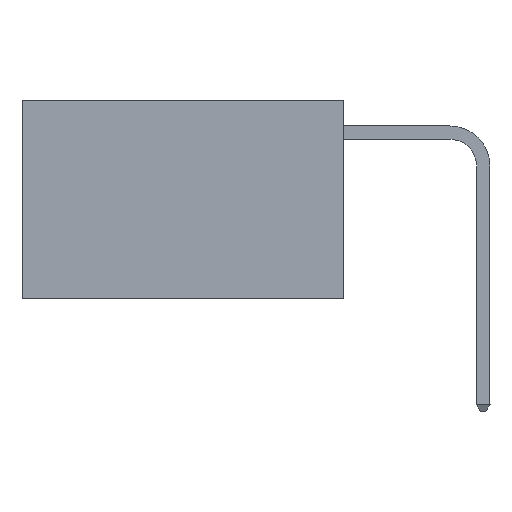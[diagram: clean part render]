
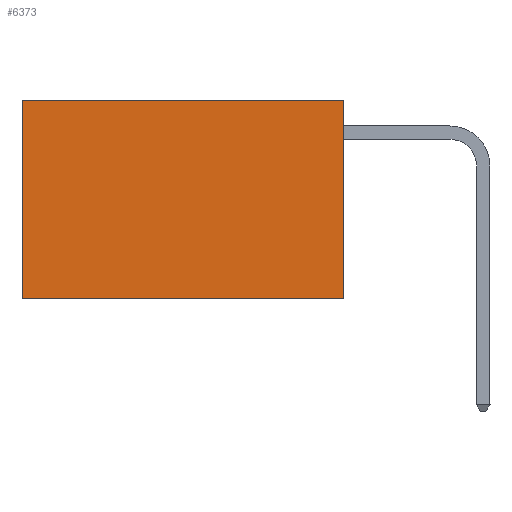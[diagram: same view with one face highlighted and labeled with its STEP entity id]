
A CAD part, left-side view. The second image highlights one B-rep face of the part: STEP entity #6373.
In plain terms, the highlighted planar face has unit normal (-1, 0, 0).
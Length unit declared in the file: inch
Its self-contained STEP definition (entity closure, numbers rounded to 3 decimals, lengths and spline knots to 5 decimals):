
#83 = ORIENTED_EDGE ( 'NONE', *, *, #4615, .T. ) ;
#137 = CARTESIAN_POINT ( 'NONE',  ( 0.2625, 0., 0. ) ) ;
#226 = CARTESIAN_POINT ( 'NONE',  ( 0.2625, 0.6, 0. ) ) ;
#648 = CARTESIAN_POINT ( 'NONE',  ( 0.2625, 0.6, 0. ) ) ;
#713 = DIRECTION ( 'NONE',  ( 0., 1., 0. ) ) ;
#1568 = DIRECTION ( 'NONE',  ( 0., 0., -1. ) ) ;
#1773 = CARTESIAN_POINT ( 'NONE',  ( 0.2625, 0., 0. ) ) ;
#3009 = AXIS2_PLACEMENT_3D ( 'NONE', #1773, #12237, #3211 ) ;
#3211 = DIRECTION ( 'NONE',  ( 0., 0., -1. ) ) ;
#3341 = LINE ( 'NONE', #137, #10021 ) ;
#4093 = VERTEX_POINT ( 'NONE', #15468 ) ;
#4615 = EDGE_CURVE ( 'NONE', #10963, #17523, #11749, .T. ) ;
#4798 = EDGE_CURVE ( 'NONE', #4093, #17523, #14006, .T. ) ;
#5026 = ORIENTED_EDGE ( 'NONE', *, *, #4798, .F. ) ;
#5235 = ORIENTED_EDGE ( 'NONE', *, *, #11759, .T. ) ;
#6373 = ADVANCED_FACE ( 'NONE', ( #18114 ), #16524, .F. ) ;
#6678 = ORIENTED_EDGE ( 'NONE', *, *, #17044, .F. ) ;
#6759 = VECTOR ( 'NONE', #1568, 39.37008 ) ;
#10021 = VECTOR ( 'NONE', #10690, 39.37008 ) ;
#10690 = DIRECTION ( 'NONE',  ( 0., 1., 0. ) ) ;
#10709 = CARTESIAN_POINT ( 'NONE',  ( 0.2625, 0., 0. ) ) ;
#10814 = VERTEX_POINT ( 'NONE', #17038 ) ;
#10963 = VERTEX_POINT ( 'NONE', #226 ) ;
#11062 = VECTOR ( 'NONE', #15085, 39.37008 ) ;
#11657 = CARTESIAN_POINT ( 'NONE',  ( 0.2625, 0.6, -0.37 ) ) ;
#11749 = LINE ( 'NONE', #648, #6759 ) ;
#11759 = EDGE_CURVE ( 'NONE', #10814, #10963, #3341, .T. ) ;
#12237 = DIRECTION ( 'NONE',  ( 1., 0., 0. ) ) ;
#13220 = EDGE_LOOP ( 'NONE', ( #83, #5026, #6678, #5235 ) ) ;
#14006 = LINE ( 'NONE', #18241, #14462 ) ;
#14462 = VECTOR ( 'NONE', #713, 39.37008 ) ;
#14919 = LINE ( 'NONE', #10709, #11062 ) ;
#15085 = DIRECTION ( 'NONE',  ( 0., 0., -1. ) ) ;
#15468 = CARTESIAN_POINT ( 'NONE',  ( 0.2625, 0., -0.37 ) ) ;
#16524 = PLANE ( 'NONE',  #3009 ) ;
#17038 = CARTESIAN_POINT ( 'NONE',  ( 0.2625, 0., 0. ) ) ;
#17044 = EDGE_CURVE ( 'NONE', #10814, #4093, #14919, .T. ) ;
#17523 = VERTEX_POINT ( 'NONE', #11657 ) ;
#18114 = FACE_OUTER_BOUND ( 'NONE', #13220, .T. ) ;
#18241 = CARTESIAN_POINT ( 'NONE',  ( 0.2625, 0., -0.37 ) ) ;
